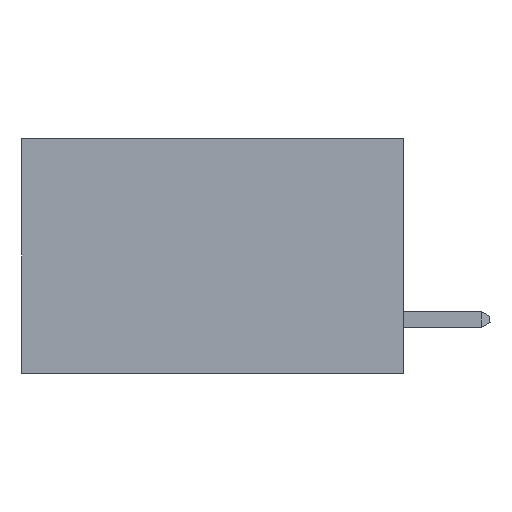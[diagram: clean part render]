
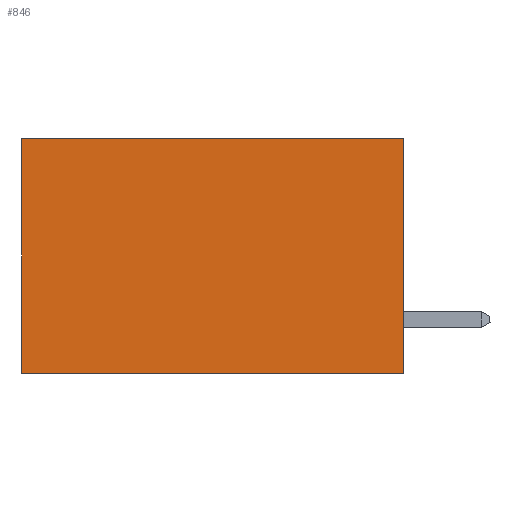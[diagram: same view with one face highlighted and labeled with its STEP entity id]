
A CAD part, left-side view. The second image highlights one B-rep face of the part: STEP entity #846.
In plain terms, the highlighted planar face has unit normal (-1, 0, 0).
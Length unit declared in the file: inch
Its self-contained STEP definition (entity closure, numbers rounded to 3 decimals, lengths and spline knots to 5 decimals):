
#366 = VERTEX_POINT ( 'NONE', #15609 ) ;
#846 = ADVANCED_FACE ( 'NONE', ( #5604 ), #10387, .F. ) ;
#1160 = CARTESIAN_POINT ( 'NONE',  ( 0.2875, 0.6, 0. ) ) ;
#2037 = VERTEX_POINT ( 'NONE', #10311 ) ;
#2932 = DIRECTION ( 'NONE',  ( 0., 0., -1. ) ) ;
#3426 = ORIENTED_EDGE ( 'NONE', *, *, #10632, .T. ) ;
#3887 = LINE ( 'NONE', #1160, #15023 ) ;
#4292 = AXIS2_PLACEMENT_3D ( 'NONE', #10287, #10418, #10474 ) ;
#4353 = CARTESIAN_POINT ( 'NONE',  ( 0.2875, 0., -0.37 ) ) ;
#5263 = VECTOR ( 'NONE', #10684, 39.37008 ) ;
#5604 = FACE_OUTER_BOUND ( 'NONE', #26058, .T. ) ;
#6375 = DIRECTION ( 'NONE',  ( 0., 1., 0. ) ) ;
#7178 = ORIENTED_EDGE ( 'NONE', *, *, #11530, .T. ) ;
#7334 = EDGE_CURVE ( 'NONE', #366, #7766, #13938, .T. ) ;
#7724 = CARTESIAN_POINT ( 'NONE',  ( 0.2875, 0.6, -0.37 ) ) ;
#7766 = VERTEX_POINT ( 'NONE', #7724 ) ;
#8655 = CARTESIAN_POINT ( 'NONE',  ( 0.2875, 0., 0. ) ) ;
#10220 = LINE ( 'NONE', #23029, #5263 ) ;
#10287 = CARTESIAN_POINT ( 'NONE',  ( 0.2875, 0., 0. ) ) ;
#10311 = CARTESIAN_POINT ( 'NONE',  ( 0.2875, 0.6, 0. ) ) ;
#10387 = PLANE ( 'NONE',  #4292 ) ;
#10418 = DIRECTION ( 'NONE',  ( 1., 0., 0. ) ) ;
#10474 = DIRECTION ( 'NONE',  ( 0., 0., -1. ) ) ;
#10632 = EDGE_CURVE ( 'NONE', #16412, #2037, #10220, .T. ) ;
#10684 = DIRECTION ( 'NONE',  ( 0., 1., 0. ) ) ;
#11028 = LINE ( 'NONE', #17562, #15860 ) ;
#11530 = EDGE_CURVE ( 'NONE', #2037, #7766, #3887, .T. ) ;
#13794 = DIRECTION ( 'NONE',  ( 0., 0., -1. ) ) ;
#13920 = ORIENTED_EDGE ( 'NONE', *, *, #21926, .F. ) ;
#13938 = LINE ( 'NONE', #4353, #19418 ) ;
#15023 = VECTOR ( 'NONE', #13794, 39.37008 ) ;
#15609 = CARTESIAN_POINT ( 'NONE',  ( 0.2875, 0., -0.37 ) ) ;
#15860 = VECTOR ( 'NONE', #2932, 39.37008 ) ;
#16412 = VERTEX_POINT ( 'NONE', #8655 ) ;
#17562 = CARTESIAN_POINT ( 'NONE',  ( 0.2875, 0., 0. ) ) ;
#19418 = VECTOR ( 'NONE', #6375, 39.37008 ) ;
#19658 = ORIENTED_EDGE ( 'NONE', *, *, #7334, .F. ) ;
#21926 = EDGE_CURVE ( 'NONE', #16412, #366, #11028, .T. ) ;
#23029 = CARTESIAN_POINT ( 'NONE',  ( 0.2875, 0., 0. ) ) ;
#26058 = EDGE_LOOP ( 'NONE', ( #7178, #19658, #13920, #3426 ) ) ;
